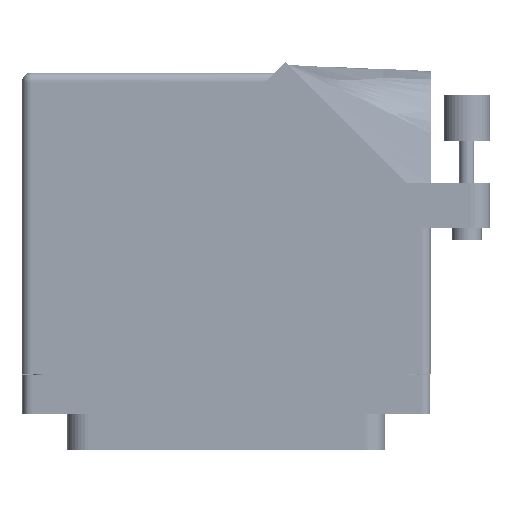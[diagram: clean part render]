
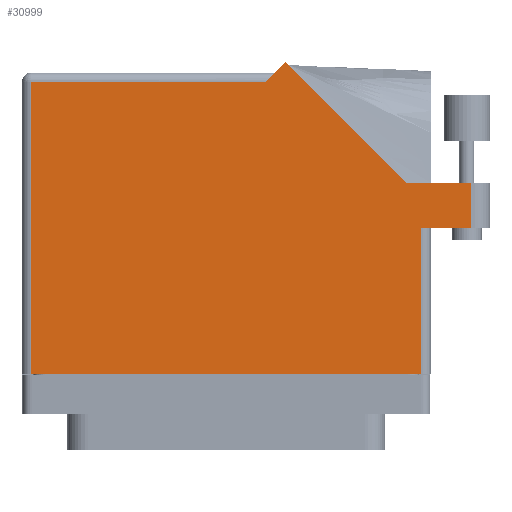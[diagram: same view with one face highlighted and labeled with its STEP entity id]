
A CAD part, front view. The second image highlights one B-rep face of the part: STEP entity #30999.
In plain terms, the highlighted face is planar.
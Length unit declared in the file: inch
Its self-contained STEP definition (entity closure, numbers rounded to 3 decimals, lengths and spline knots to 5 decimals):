
#931 = DIRECTION ( 'NONE',  ( 1., 0., 0. ) ) ;
#1005 = ORIENTED_EDGE ( 'NONE', *, *, #5602, .T. ) ;
#1220 = ORIENTED_EDGE ( 'NONE', *, *, #38024, .T. ) ;
#2208 = DIRECTION ( 'NONE',  ( -1., 0., 0. ) ) ;
#3137 = VECTOR ( 'NONE', #22919, 39.37008 ) ;
#3992 = CARTESIAN_POINT ( 'NONE',  ( -1.3155, -0.1, 0.765 ) ) ;
#5505 = CARTESIAN_POINT ( 'NONE',  ( 0.2655, 1.868, 0.765 ) ) ;
#5602 = EDGE_CURVE ( 'NONE', #32893, #8900, #11733, .T. ) ;
#5750 = CARTESIAN_POINT ( 'NONE',  ( 0.39821, 2.00071, 0.765 ) ) ;
#6407 = PLANE ( 'NONE',  #62368 ) ;
#6647 = EDGE_CURVE ( 'NONE', #76331, #27856, #58593, .T. ) ;
#7323 = DIRECTION ( 'NONE',  ( -1., 0., 0. ) ) ;
#8900 = VERTEX_POINT ( 'NONE', #83840 ) ;
#8919 = ORIENTED_EDGE ( 'NONE', *, *, #22902, .T. ) ;
#8942 = DIRECTION ( 'NONE',  ( -0.707, 0.707, 0. ) ) ;
#9894 = ORIENTED_EDGE ( 'NONE', *, *, #6647, .T. ) ;
#11079 = LINE ( 'NONE', #54313, #42414 ) ;
#11522 = ORIENTED_EDGE ( 'NONE', *, *, #64641, .T. ) ;
#11733 = LINE ( 'NONE', #46115, #55433 ) ;
#12160 = CARTESIAN_POINT ( 'NONE',  ( 1.3155, 0.88, 0.765 ) ) ;
#16488 = CARTESIAN_POINT ( 'NONE',  ( 1.21192, 1.187, 0.765 ) ) ;
#19173 = DIRECTION ( 'NONE',  ( -1., 0., 0. ) ) ;
#19806 = ORIENTED_EDGE ( 'NONE', *, *, #72442, .T. ) ;
#21477 = CARTESIAN_POINT ( 'NONE',  ( -1.3775, 1.93, 0.765 ) ) ;
#22902 = EDGE_CURVE ( 'NONE', #34927, #39569, #46268, .T. ) ;
#22919 = DIRECTION ( 'NONE',  ( 1., 0., 0. ) ) ;
#24074 = CARTESIAN_POINT ( 'NONE',  ( 1.21192, 1.187, 0.765 ) ) ;
#26442 = CARTESIAN_POINT ( 'NONE',  ( 1.7775, 1.187, 0.765 ) ) ;
#27837 = EDGE_CURVE ( 'NONE', #8900, #34927, #74648, .T. ) ;
#27856 = VERTEX_POINT ( 'NONE', #5750 ) ;
#28331 = DIRECTION ( 'NONE',  ( 0., -1., 0. ) ) ;
#30999 = ADVANCED_FACE ( 'NONE', ( #76252 ), #6407, .F. ) ;
#31541 = ORIENTED_EDGE ( 'NONE', *, *, #27837, .T. ) ;
#32893 = VERTEX_POINT ( 'NONE', #5505 ) ;
#33734 = LINE ( 'NONE', #26442, #51674 ) ;
#34420 = ORIENTED_EDGE ( 'NONE', *, *, #79985, .T. ) ;
#34528 = CARTESIAN_POINT ( 'NONE',  ( -1.3155, -0.1, 0.765 ) ) ;
#34927 = VERTEX_POINT ( 'NONE', #3992 ) ;
#38024 = EDGE_CURVE ( 'NONE', #84238, #76331, #33734, .T. ) ;
#38867 = VERTEX_POINT ( 'NONE', #12160 ) ;
#39569 = VERTEX_POINT ( 'NONE', #72333 ) ;
#39877 = CARTESIAN_POINT ( 'NONE',  ( 1.6525, 0.88, 0.765 ) ) ;
#40016 = VERTEX_POINT ( 'NONE', #39877 ) ;
#42414 = VECTOR ( 'NONE', #82587, 39.37008 ) ;
#46013 = CARTESIAN_POINT ( 'NONE',  ( 1.3155, 0.88, 0.765 ) ) ;
#46115 = CARTESIAN_POINT ( 'NONE',  ( -1.3775, 1.868, 0.765 ) ) ;
#46268 = LINE ( 'NONE', #58283, #70922 ) ;
#48304 = LINE ( 'NONE', #73051, #70707 ) ;
#49020 = ORIENTED_EDGE ( 'NONE', *, *, #91477, .T. ) ;
#49635 = VECTOR ( 'NONE', #8942, 39.37008 ) ;
#50231 = DIRECTION ( 'NONE',  ( 0., 0., -1. ) ) ;
#51674 = VECTOR ( 'NONE', #19173, 39.37008 ) ;
#52085 = VECTOR ( 'NONE', #28331, 39.37008 ) ;
#53907 = VECTOR ( 'NONE', #73323, 39.37008 ) ;
#54313 = CARTESIAN_POINT ( 'NONE',  ( 1.6525, 1.187, 0.765 ) ) ;
#55433 = VECTOR ( 'NONE', #2208, 39.37008 ) ;
#58283 = CARTESIAN_POINT ( 'NONE',  ( -1.3775, -0.1, 0.765 ) ) ;
#58541 = CARTESIAN_POINT ( 'NONE',  ( 1.3775, 0.88, 0.765 ) ) ;
#58593 = LINE ( 'NONE', #24074, #49635 ) ;
#62368 = AXIS2_PLACEMENT_3D ( 'NONE', #21477, #50231, #7323 ) ;
#64641 = EDGE_CURVE ( 'NONE', #38867, #40016, #67103, .T. ) ;
#67103 = LINE ( 'NONE', #58541, #3137 ) ;
#68483 = LINE ( 'NONE', #46013, #53907 ) ;
#70707 = VECTOR ( 'NONE', #80898, 39.37008 ) ;
#70922 = VECTOR ( 'NONE', #931, 39.37008 ) ;
#72333 = CARTESIAN_POINT ( 'NONE',  ( 1.3155, -0.1, 0.765 ) ) ;
#72442 = EDGE_CURVE ( 'NONE', #39569, #38867, #68483, .T. ) ;
#73051 = CARTESIAN_POINT ( 'NONE',  ( 0.3275, 1.93, 0.765 ) ) ;
#73323 = DIRECTION ( 'NONE',  ( 0., 1., 0. ) ) ;
#74648 = LINE ( 'NONE', #34528, #52085 ) ;
#76252 = FACE_OUTER_BOUND ( 'NONE', #90534, .T. ) ;
#76331 = VERTEX_POINT ( 'NONE', #16488 ) ;
#79985 = EDGE_CURVE ( 'NONE', #40016, #84238, #11079, .T. ) ;
#80807 = CARTESIAN_POINT ( 'NONE',  ( 1.6525, 1.187, 0.765 ) ) ;
#80898 = DIRECTION ( 'NONE',  ( -0.707, -0.707, 0. ) ) ;
#82587 = DIRECTION ( 'NONE',  ( 0., 1., 0. ) ) ;
#83840 = CARTESIAN_POINT ( 'NONE',  ( -1.3155, 1.868, 0.765 ) ) ;
#84238 = VERTEX_POINT ( 'NONE', #80807 ) ;
#90534 = EDGE_LOOP ( 'NONE', ( #11522, #34420, #1220, #9894, #49020, #1005, #31541, #8919, #19806 ) ) ;
#91477 = EDGE_CURVE ( 'NONE', #27856, #32893, #48304, .T. ) ;
